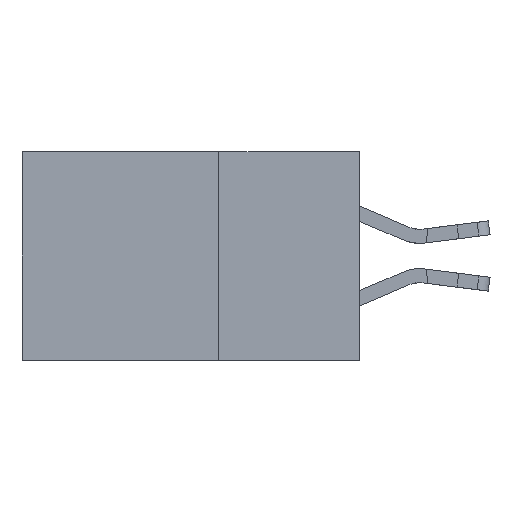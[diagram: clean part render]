
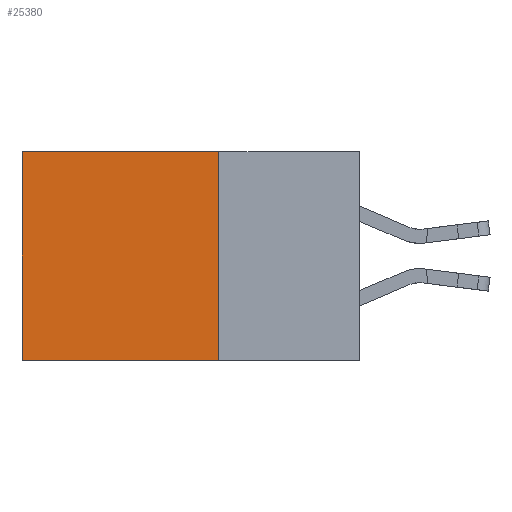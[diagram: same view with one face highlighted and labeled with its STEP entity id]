
A CAD part, left-side view. The second image highlights one B-rep face of the part: STEP entity #25380.
In plain terms, the highlighted planar face has unit normal (-1, 0, 0).
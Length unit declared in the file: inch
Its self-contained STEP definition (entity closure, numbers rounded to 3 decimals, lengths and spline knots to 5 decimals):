
#172 = CARTESIAN_POINT ( 'NONE',  ( 0.2875, 0.6, 0. ) ) ;
#2651 = VERTEX_POINT ( 'NONE', #27545 ) ;
#3472 = CARTESIAN_POINT ( 'NONE',  ( 0.2875, 0.25, 0. ) ) ;
#4484 = LINE ( 'NONE', #5056, #10014 ) ;
#5056 = CARTESIAN_POINT ( 'NONE',  ( 0.2875, 0.25, -0.37 ) ) ;
#5063 = EDGE_LOOP ( 'NONE', ( #12827, #32419, #25570, #8995 ) ) ;
#7629 = VECTOR ( 'NONE', #14548, 39.37008 ) ;
#8995 = ORIENTED_EDGE ( 'NONE', *, *, #11387, .T. ) ;
#9618 = CARTESIAN_POINT ( 'NONE',  ( 0.2875, 0.25, 0. ) ) ;
#9847 = EDGE_CURVE ( 'NONE', #26723, #17115, #27605, .T. ) ;
#10014 = VECTOR ( 'NONE', #13619, 39.37008 ) ;
#11387 = EDGE_CURVE ( 'NONE', #11572, #26723, #32915, .T. ) ;
#11572 = VERTEX_POINT ( 'NONE', #12346 ) ;
#11681 = DIRECTION ( 'NONE',  ( 0., 1., 0. ) ) ;
#12346 = CARTESIAN_POINT ( 'NONE',  ( 0.2875, 0.25, 0. ) ) ;
#12827 = ORIENTED_EDGE ( 'NONE', *, *, #9847, .T. ) ;
#13530 = CARTESIAN_POINT ( 'NONE',  ( 0.2875, 0.6, -0.37 ) ) ;
#13619 = DIRECTION ( 'NONE',  ( 0., 1., 0. ) ) ;
#14548 = DIRECTION ( 'NONE',  ( 0., 0., -1. ) ) ;
#14783 = CARTESIAN_POINT ( 'NONE',  ( 0.2875, 0.6, 0. ) ) ;
#15082 = VECTOR ( 'NONE', #11681, 39.37008 ) ;
#16863 = CARTESIAN_POINT ( 'NONE',  ( 0.2875, 0.25, 0. ) ) ;
#17103 = PLANE ( 'NONE',  #20192 ) ;
#17115 = VERTEX_POINT ( 'NONE', #13530 ) ;
#17636 = LINE ( 'NONE', #9618, #18019 ) ;
#18019 = VECTOR ( 'NONE', #18064, 39.37008 ) ;
#18064 = DIRECTION ( 'NONE',  ( 0., 0., -1. ) ) ;
#18633 = FACE_OUTER_BOUND ( 'NONE', #5063, .T. ) ;
#20192 = AXIS2_PLACEMENT_3D ( 'NONE', #16863, #27890, #22311 ) ;
#20378 = EDGE_CURVE ( 'NONE', #11572, #2651, #17636, .T. ) ;
#22311 = DIRECTION ( 'NONE',  ( 0., 0., -1. ) ) ;
#25380 = ADVANCED_FACE ( 'NONE', ( #18633 ), #17103, .F. ) ;
#25570 = ORIENTED_EDGE ( 'NONE', *, *, #20378, .F. ) ;
#26723 = VERTEX_POINT ( 'NONE', #172 ) ;
#27545 = CARTESIAN_POINT ( 'NONE',  ( 0.2875, 0.25, -0.37 ) ) ;
#27605 = LINE ( 'NONE', #14783, #7629 ) ;
#27890 = DIRECTION ( 'NONE',  ( 1., 0., 0. ) ) ;
#32419 = ORIENTED_EDGE ( 'NONE', *, *, #33101, .F. ) ;
#32915 = LINE ( 'NONE', #3472, #15082 ) ;
#33101 = EDGE_CURVE ( 'NONE', #2651, #17115, #4484, .T. ) ;
